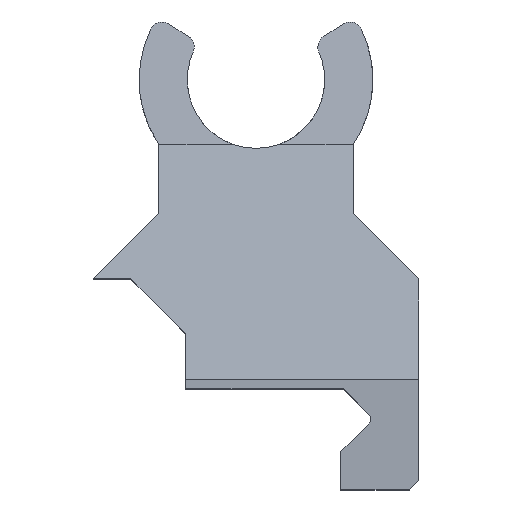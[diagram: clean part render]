
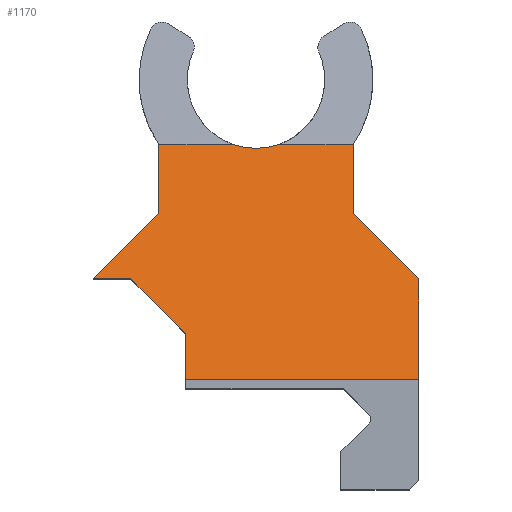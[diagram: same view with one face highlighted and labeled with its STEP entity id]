
A CAD part, top view. The second image highlights one B-rep face of the part: STEP entity #1170.
In plain terms, the highlighted planar face has unit normal (0, 0.281, 0.96).
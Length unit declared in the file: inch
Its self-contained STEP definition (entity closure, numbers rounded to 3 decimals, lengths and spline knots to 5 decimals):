
#2 = VECTOR ( 'NONE', #3279, 39.37008 ) ;
#33 = CARTESIAN_POINT ( 'NONE',  ( -0.5925, 0.14418, 0.6 ) ) ;
#64 = DIRECTION ( 'NONE',  ( 0., -0.281, -0.96 ) ) ;
#129 = DIRECTION ( 'NONE',  ( 0.692, 0.692, -0.203 ) ) ;
#146 = DIRECTION ( 'NONE',  ( 1., 0., 0. ) ) ;
#157 = LINE ( 'NONE', #2349, #2 ) ;
#194 = VECTOR ( 'NONE', #146, 39.37008 ) ;
#215 = FACE_OUTER_BOUND ( 'NONE', #2440, .T. ) ;
#262 = VERTEX_POINT ( 'NONE', #3164 ) ;
#263 = ORIENTED_EDGE ( 'NONE', *, *, #1828, .F. ) ;
#280 = ORIENTED_EDGE ( 'NONE', *, *, #503, .F. ) ;
#316 = CARTESIAN_POINT ( 'NONE',  ( -0.36218, 0.41693, 0.52023 ) ) ;
#329 = DIRECTION ( 'NONE',  ( 0., -0.96, 0.281 ) ) ;
#370 = CARTESIAN_POINT ( 'NONE',  ( -0.5925, 0.51, 0.49302 ) ) ;
#371 = VECTOR ( 'NONE', #2270, 39.37008 ) ;
#376 = CARTESIAN_POINT ( 'NONE',  ( -0.08257, 0.99903, 0.35 ) ) ;
#440 = CARTESIAN_POINT ( 'NONE',  ( -0.25525, 0.14418, 0.6 ) ) ;
#503 = EDGE_CURVE ( 'NONE', #2313, #2176, #3501, .T. ) ;
#552 = DIRECTION ( 'NONE',  ( 0.692, -0.692, 0.203 ) ) ;
#569 = VERTEX_POINT ( 'NONE', #3616 ) ;
#588 = DIRECTION ( 'NONE',  ( 0., -0.96, 0.281 ) ) ;
#633 = EDGE_CURVE ( 'NONE', #3852, #2628, #2117, .T. ) ;
#639 = LINE ( 'NONE', #1521, #2539 ) ;
#824 = CARTESIAN_POINT ( 'NONE',  ( 0.5925, 0.51, 0.49302 ) ) ;
#902 = LINE ( 'NONE', #3515, #2587 ) ;
#991 = DIRECTION ( 'NONE',  ( 0., 0.96, -0.281 ) ) ;
#1018 = CARTESIAN_POINT ( 'NONE',  ( -0.35347, 0.74903, 0.42311 ) ) ;
#1057 = LINE ( 'NONE', #1104, #2892 ) ;
#1104 = CARTESIAN_POINT ( 'NONE',  ( -0.6075, 0.495, 0.4974 ) ) ;
#1112 = CARTESIAN_POINT ( 'NONE',  ( 0.02859, 0.98014, 0.35552 ) ) ;
#1125 = CARTESIAN_POINT ( 'NONE',  ( -0.25525, 0.31, 0.55151 ) ) ;
#1165 = LINE ( 'NONE', #316, #4145 ) ;
#1170 = ADVANCED_FACE ( 'NONE', ( #215 ), #3295, .F. ) ;
#1196 = CARTESIAN_POINT ( 'NONE',  ( 0.5925, 0.14418, 0.6 ) ) ;
#1446 = CARTESIAN_POINT ( 'NONE',  ( 0.08257, 0.99903, 0.35 ) ) ;
#1457 = VERTEX_POINT ( 'NONE', #824 ) ;
#1485 = CARTESIAN_POINT ( 'NONE',  ( 0.6075, 0.495, 0.4974 ) ) ;
#1521 = CARTESIAN_POINT ( 'NONE',  ( -0.5925, 0.99903, 0.35 ) ) ;
#1550 = DIRECTION ( 'NONE',  ( 0., 0.96, -0.281 ) ) ;
#1588 = LINE ( 'NONE', #1485, #2858 ) ;
#1629 = DIRECTION ( 'NONE',  ( 0.692, -0.692, 0.203 ) ) ;
#1655 = VECTOR ( 'NONE', #329, 39.37008 ) ;
#1726 = DIRECTION ( 'NONE',  ( 0., 0.96, -0.281 ) ) ;
#1737 = ORIENTED_EDGE ( 'NONE', *, *, #2609, .F. ) ;
#1794 = ORIENTED_EDGE ( 'NONE', *, *, #4097, .F. ) ;
#1809 = AXIS2_PLACEMENT_3D ( 'NONE', #3972, #64, #991 ) ;
#1828 = EDGE_CURVE ( 'NONE', #569, #2399, #157, .T. ) ;
#1878 = ORIENTED_EDGE ( 'NONE', *, *, #633, .T. ) ;
#1952 = ORIENTED_EDGE ( 'NONE', *, *, #2153, .F. ) ;
#2039 = VERTEX_POINT ( 'NONE', #1125 ) ;
#2117 = LINE ( 'NONE', #33, #371 ) ;
#2153 = EDGE_CURVE ( 'NONE', #2351, #262, #3537, .T. ) ;
#2176 = VERTEX_POINT ( 'NONE', #4036 ) ;
#2209 = VERTEX_POINT ( 'NONE', #4055 ) ;
#2270 = DIRECTION ( 'NONE',  ( 1., 0., 0. ) ) ;
#2291 =( BOUNDED_CURVE ( )  B_SPLINE_CURVE ( 3, ( #2741, #3069, #1112, #1446 ),
 .UNSPECIFIED., .F., .T. ) 
 B_SPLINE_CURVE_WITH_KNOTS ( ( 4, 4 ),
 ( 2.80501, 3.47818 ),
 .UNSPECIFIED. ) 
 CURVE ( )  GEOMETRIC_REPRESENTATION_ITEM ( )  RATIONAL_B_SPLINE_CURVE ( ( 1., 0.963, 0.963, 1. ) ) 
 REPRESENTATION_ITEM ( '' )  );
#2313 = VERTEX_POINT ( 'NONE', #2694 ) ;
#2349 = CARTESIAN_POINT ( 'NONE',  ( 0.5925, 0.51, 0.49302 ) ) ;
#2351 = VERTEX_POINT ( 'NONE', #1018 ) ;
#2399 = VERTEX_POINT ( 'NONE', #370 ) ;
#2440 = EDGE_LOOP ( 'NONE', ( #2474, #1952, #2835, #263, #4053, #1794, #1878, #2514, #1737, #280, #4202, #3073 ) ) ;
#2474 = ORIENTED_EDGE ( 'NONE', *, *, #4058, .F. ) ;
#2514 = ORIENTED_EDGE ( 'NONE', *, *, #3072, .F. ) ;
#2528 = EDGE_CURVE ( 'NONE', #2880, #2209, #2291, .T. ) ;
#2539 = VECTOR ( 'NONE', #3810, 39.37008 ) ;
#2542 = CARTESIAN_POINT ( 'NONE',  ( 0.5925, -0.19282, 0.69856 ) ) ;
#2587 = VECTOR ( 'NONE', #1550, 39.37008 ) ;
#2609 = EDGE_CURVE ( 'NONE', #2176, #1457, #1588, .T. ) ;
#2628 = VERTEX_POINT ( 'NONE', #1196 ) ;
#2694 = CARTESIAN_POINT ( 'NONE',  ( 0.35347, 0.99903, 0.35 ) ) ;
#2699 = LINE ( 'NONE', #2542, #2852 ) ;
#2741 = CARTESIAN_POINT ( 'NONE',  ( -0.08257, 0.99903, 0.35 ) ) ;
#2835 = ORIENTED_EDGE ( 'NONE', *, *, #3794, .F. ) ;
#2852 = VECTOR ( 'NONE', #588, 39.37008 ) ;
#2858 = VECTOR ( 'NONE', #552, 39.37008 ) ;
#2880 = VERTEX_POINT ( 'NONE', #376 ) ;
#2892 = VECTOR ( 'NONE', #129, 39.37008 ) ;
#2965 = VECTOR ( 'NONE', #1726, 39.37008 ) ;
#3069 = CARTESIAN_POINT ( 'NONE',  ( -0.02859, 0.98014, 0.35552 ) ) ;
#3072 = EDGE_CURVE ( 'NONE', #1457, #2628, #2699, .T. ) ;
#3073 = ORIENTED_EDGE ( 'NONE', *, *, #2528, .F. ) ;
#3164 = CARTESIAN_POINT ( 'NONE',  ( -0.35347, 0.99903, 0.35 ) ) ;
#3256 = LINE ( 'NONE', #4049, #194 ) ;
#3279 = DIRECTION ( 'NONE',  ( -1., 0., 0. ) ) ;
#3295 = PLANE ( 'NONE',  #1809 ) ;
#3377 = CARTESIAN_POINT ( 'NONE',  ( -0.35347, 0.93168, 0.3697 ) ) ;
#3398 = EDGE_CURVE ( 'NONE', #2209, #2313, #3256, .T. ) ;
#3501 = LINE ( 'NONE', #3932, #1655 ) ;
#3515 = CARTESIAN_POINT ( 'NONE',  ( -0.25525, 0.29694, 0.55533 ) ) ;
#3537 = LINE ( 'NONE', #3377, #2965 ) ;
#3572 = EDGE_CURVE ( 'NONE', #569, #2039, #1165, .T. ) ;
#3616 = CARTESIAN_POINT ( 'NONE',  ( -0.45525, 0.51, 0.49302 ) ) ;
#3794 = EDGE_CURVE ( 'NONE', #2399, #2351, #1057, .T. ) ;
#3810 = DIRECTION ( 'NONE',  ( 1., 0., 0. ) ) ;
#3852 = VERTEX_POINT ( 'NONE', #440 ) ;
#3932 = CARTESIAN_POINT ( 'NONE',  ( 0.35347, 0.93168, 0.3697 ) ) ;
#3972 = CARTESIAN_POINT ( 'NONE',  ( -0.5925, 0.99903, 0.35 ) ) ;
#4036 = CARTESIAN_POINT ( 'NONE',  ( 0.35347, 0.74903, 0.42311 ) ) ;
#4049 = CARTESIAN_POINT ( 'NONE',  ( -0.5925, 0.99903, 0.35 ) ) ;
#4053 = ORIENTED_EDGE ( 'NONE', *, *, #3572, .T. ) ;
#4055 = CARTESIAN_POINT ( 'NONE',  ( 0.08257, 0.99903, 0.35 ) ) ;
#4058 = EDGE_CURVE ( 'NONE', #262, #2880, #639, .T. ) ;
#4097 = EDGE_CURVE ( 'NONE', #3852, #2039, #902, .T. ) ;
#4145 = VECTOR ( 'NONE', #1629, 39.37008 ) ;
#4202 = ORIENTED_EDGE ( 'NONE', *, *, #3398, .F. ) ;
